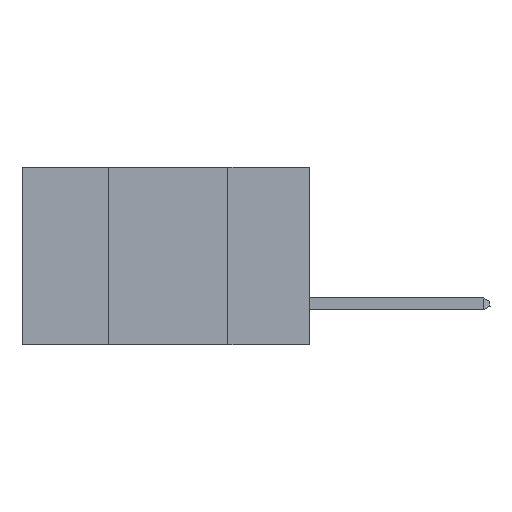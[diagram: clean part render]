
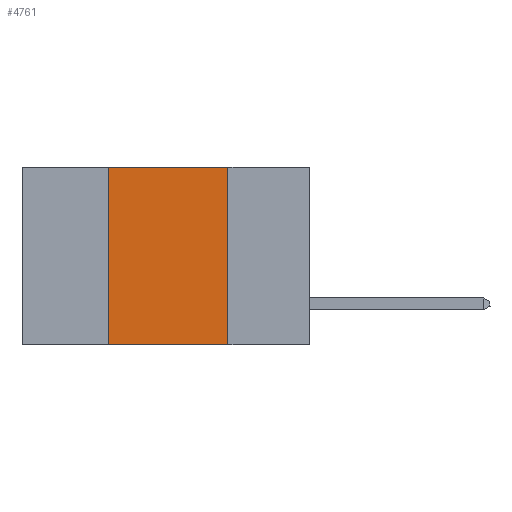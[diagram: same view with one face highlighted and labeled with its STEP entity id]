
A CAD part, left-side view. The second image highlights one B-rep face of the part: STEP entity #4761.
In plain terms, the highlighted planar face has unit normal (-1, 0, 0).
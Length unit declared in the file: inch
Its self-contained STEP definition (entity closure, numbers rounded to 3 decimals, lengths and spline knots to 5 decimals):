
#727 = VERTEX_POINT ( 'NONE', #9800 ) ;
#1167 = ORIENTED_EDGE ( 'NONE', *, *, #7795, .F. ) ;
#1744 = DIRECTION ( 'NONE',  ( 1., 0., 0. ) ) ;
#2629 = CARTESIAN_POINT ( 'NONE',  ( 0., 0.42, -0.37 ) ) ;
#2958 = CARTESIAN_POINT ( 'NONE',  ( 0., 0.6, 0. ) ) ;
#2985 = CARTESIAN_POINT ( 'NONE',  ( 0., 0.17, -0.37 ) ) ;
#3338 = ORIENTED_EDGE ( 'NONE', *, *, #10588, .F. ) ;
#3410 = EDGE_CURVE ( 'NONE', #14348, #727, #11844, .T. ) ;
#3578 = VERTEX_POINT ( 'NONE', #2629 ) ;
#3801 = CARTESIAN_POINT ( 'NONE',  ( 0., 0.42, 0. ) ) ;
#4167 = DIRECTION ( 'NONE',  ( 0., 0., -1. ) ) ;
#4537 = DIRECTION ( 'NONE',  ( 0., 0., -1. ) ) ;
#4607 = VECTOR ( 'NONE', #12567, 39.37008 ) ;
#4701 = DIRECTION ( 'NONE',  ( 0., -1., 0. ) ) ;
#4761 = ADVANCED_FACE ( 'NONE', ( #4914 ), #13856, .F. ) ;
#4914 = FACE_OUTER_BOUND ( 'NONE', #9685, .T. ) ;
#6254 = ORIENTED_EDGE ( 'NONE', *, *, #3410, .F. ) ;
#6457 = LINE ( 'NONE', #10724, #14625 ) ;
#6639 = VECTOR ( 'NONE', #4537, 39.37008 ) ;
#7745 = CARTESIAN_POINT ( 'NONE',  ( 0., 0.6, 0. ) ) ;
#7795 = EDGE_CURVE ( 'NONE', #3578, #14348, #8861, .T. ) ;
#8716 = AXIS2_PLACEMENT_3D ( 'NONE', #7745, #1744, #4167 ) ;
#8773 = VERTEX_POINT ( 'NONE', #2985 ) ;
#8861 = LINE ( 'NONE', #3801, #14735 ) ;
#9685 = EDGE_LOOP ( 'NONE', ( #3338, #6254, #1167, #15536 ) ) ;
#9800 = CARTESIAN_POINT ( 'NONE',  ( 0., 0.17, 0. ) ) ;
#10588 = EDGE_CURVE ( 'NONE', #727, #8773, #10681, .T. ) ;
#10653 = EDGE_CURVE ( 'NONE', #3578, #8773, #6457, .T. ) ;
#10681 = LINE ( 'NONE', #11715, #6639 ) ;
#10724 = CARTESIAN_POINT ( 'NONE',  ( 0., 0.6, -0.37 ) ) ;
#11715 = CARTESIAN_POINT ( 'NONE',  ( 0., 0.17, 0. ) ) ;
#11844 = LINE ( 'NONE', #2958, #4607 ) ;
#11884 = CARTESIAN_POINT ( 'NONE',  ( 0., 0.42, 0. ) ) ;
#12567 = DIRECTION ( 'NONE',  ( 0., -1., 0. ) ) ;
#12880 = DIRECTION ( 'NONE',  ( 0., 0., 1. ) ) ;
#13856 = PLANE ( 'NONE',  #8716 ) ;
#14348 = VERTEX_POINT ( 'NONE', #11884 ) ;
#14625 = VECTOR ( 'NONE', #4701, 39.37008 ) ;
#14735 = VECTOR ( 'NONE', #12880, 39.37008 ) ;
#15536 = ORIENTED_EDGE ( 'NONE', *, *, #10653, .T. ) ;
